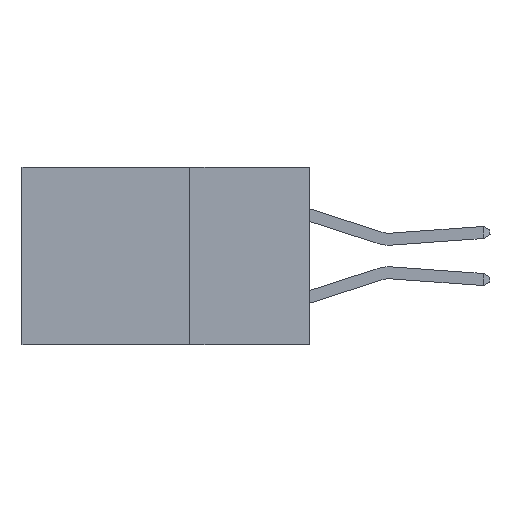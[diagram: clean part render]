
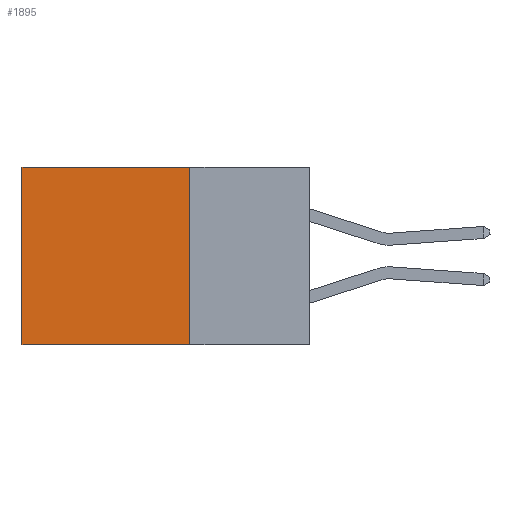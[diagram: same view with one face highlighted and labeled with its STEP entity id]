
A CAD part, left-side view. The second image highlights one B-rep face of the part: STEP entity #1895.
In plain terms, the highlighted planar face has unit normal (-1, 0, 0).
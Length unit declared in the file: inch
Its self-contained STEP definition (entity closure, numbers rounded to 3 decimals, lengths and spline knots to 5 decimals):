
#781 = VECTOR ( 'NONE', #14192, 39.37008 ) ;
#972 = VERTEX_POINT ( 'NONE', #9915 ) ;
#1558 = CARTESIAN_POINT ( 'NONE',  ( 0.2615, 0.25, -0.37 ) ) ;
#1563 = CARTESIAN_POINT ( 'NONE',  ( 0.2615, 0.25, -0.37 ) ) ;
#1895 = ADVANCED_FACE ( 'NONE', ( #4609 ), #11708, .F. ) ;
#3037 = DIRECTION ( 'NONE',  ( 0., 0., -1. ) ) ;
#3801 = VECTOR ( 'NONE', #13447, 39.37008 ) ;
#3871 = CARTESIAN_POINT ( 'NONE',  ( 0.2615, 0.6, -0.37 ) ) ;
#3913 = ORIENTED_EDGE ( 'NONE', *, *, #13202, .T. ) ;
#4439 = DIRECTION ( 'NONE',  ( 1., 0., 0. ) ) ;
#4609 = FACE_OUTER_BOUND ( 'NONE', #12459, .T. ) ;
#4974 = VECTOR ( 'NONE', #3037, 39.37008 ) ;
#5252 = EDGE_CURVE ( 'NONE', #6461, #13300, #8315, .T. ) ;
#5549 = ORIENTED_EDGE ( 'NONE', *, *, #5252, .T. ) ;
#5617 = CARTESIAN_POINT ( 'NONE',  ( 0.2615, 0.6, -0.37 ) ) ;
#6249 = EDGE_CURVE ( 'NONE', #972, #13158, #10117, .T. ) ;
#6461 = VERTEX_POINT ( 'NONE', #15882 ) ;
#6994 = EDGE_CURVE ( 'NONE', #13158, #13300, #9250, .T. ) ;
#8315 = LINE ( 'NONE', #5617, #781 ) ;
#9195 = AXIS2_PLACEMENT_3D ( 'NONE', #1563, #4439, #17305 ) ;
#9250 = LINE ( 'NONE', #13815, #3801 ) ;
#9362 = DIRECTION ( 'NONE',  ( 0., 1., 0. ) ) ;
#9915 = CARTESIAN_POINT ( 'NONE',  ( 0.2615, 0.25, 0. ) ) ;
#10117 = LINE ( 'NONE', #11430, #4974 ) ;
#11430 = CARTESIAN_POINT ( 'NONE',  ( 0.2615, 0.25, -0.37 ) ) ;
#11629 = VECTOR ( 'NONE', #9362, 39.37008 ) ;
#11708 = PLANE ( 'NONE',  #9195 ) ;
#11975 = CARTESIAN_POINT ( 'NONE',  ( 0.2615, 0.25, 0. ) ) ;
#12459 = EDGE_LOOP ( 'NONE', ( #5549, #14092, #17287, #3913 ) ) ;
#13158 = VERTEX_POINT ( 'NONE', #1558 ) ;
#13202 = EDGE_CURVE ( 'NONE', #972, #6461, #16355, .T. ) ;
#13300 = VERTEX_POINT ( 'NONE', #3871 ) ;
#13447 = DIRECTION ( 'NONE',  ( 0., 1., 0. ) ) ;
#13815 = CARTESIAN_POINT ( 'NONE',  ( 0.2615, 0.25, -0.37 ) ) ;
#14092 = ORIENTED_EDGE ( 'NONE', *, *, #6994, .F. ) ;
#14192 = DIRECTION ( 'NONE',  ( 0., 0., -1. ) ) ;
#15882 = CARTESIAN_POINT ( 'NONE',  ( 0.2615, 0.6, 0. ) ) ;
#16355 = LINE ( 'NONE', #11975, #11629 ) ;
#17287 = ORIENTED_EDGE ( 'NONE', *, *, #6249, .F. ) ;
#17305 = DIRECTION ( 'NONE',  ( 0., 0., -1. ) ) ;
